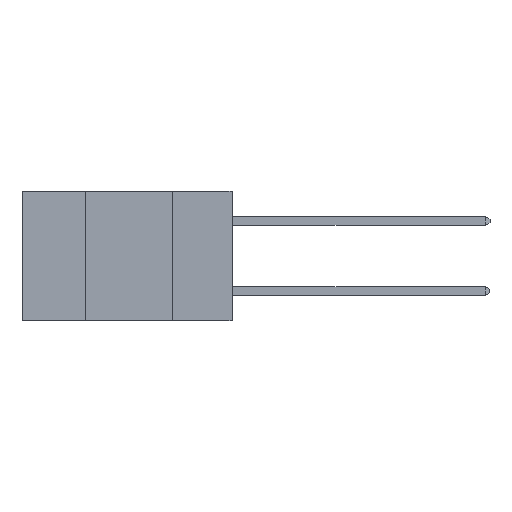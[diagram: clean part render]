
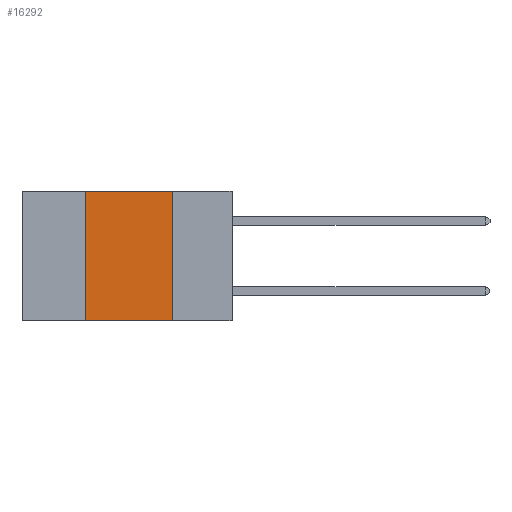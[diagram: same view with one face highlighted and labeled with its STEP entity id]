
A CAD part, left-side view. The second image highlights one B-rep face of the part: STEP entity #16292.
In plain terms, the highlighted planar face has unit normal (-1, 0, 0).
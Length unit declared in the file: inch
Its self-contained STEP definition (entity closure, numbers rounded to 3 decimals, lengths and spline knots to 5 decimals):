
#39 = CARTESIAN_POINT ( 'NONE',  ( 0., 0.17, 0. ) ) ;
#438 = FACE_OUTER_BOUND ( 'NONE', #10983, .T. ) ;
#834 = EDGE_CURVE ( 'NONE', #3131, #1718, #4436, .T. ) ;
#1718 = VERTEX_POINT ( 'NONE', #2014 ) ;
#2014 = CARTESIAN_POINT ( 'NONE',  ( 0., 0.17, -0.37 ) ) ;
#2199 = CARTESIAN_POINT ( 'NONE',  ( 0., 0.6, 0. ) ) ;
#3131 = VERTEX_POINT ( 'NONE', #10765 ) ;
#3248 = CARTESIAN_POINT ( 'NONE',  ( 0., 0.6, -0.37 ) ) ;
#3613 = DIRECTION ( 'NONE',  ( 0., 0., -1. ) ) ;
#3920 = VERTEX_POINT ( 'NONE', #12405 ) ;
#4272 = CARTESIAN_POINT ( 'NONE',  ( 0., 0.42, 0. ) ) ;
#4436 = LINE ( 'NONE', #3248, #14117 ) ;
#5239 = ORIENTED_EDGE ( 'NONE', *, *, #14721, .F. ) ;
#5408 = ORIENTED_EDGE ( 'NONE', *, *, #7624, .F. ) ;
#5524 = ORIENTED_EDGE ( 'NONE', *, *, #10147, .F. ) ;
#5672 = LINE ( 'NONE', #13204, #11907 ) ;
#5674 = DIRECTION ( 'NONE',  ( 0., 0., 1. ) ) ;
#5677 = ORIENTED_EDGE ( 'NONE', *, *, #834, .T. ) ;
#5875 = VECTOR ( 'NONE', #13056, 39.37008 ) ;
#7119 = LINE ( 'NONE', #4272, #13231 ) ;
#7591 = CARTESIAN_POINT ( 'NONE',  ( 0., 0.42, 0. ) ) ;
#7624 = EDGE_CURVE ( 'NONE', #15015, #3920, #5672, .T. ) ;
#8401 = AXIS2_PLACEMENT_3D ( 'NONE', #2199, #11319, #3613 ) ;
#8916 = PLANE ( 'NONE',  #8401 ) ;
#9879 = DIRECTION ( 'NONE',  ( 0., -1., 0. ) ) ;
#10147 = EDGE_CURVE ( 'NONE', #3131, #15015, #7119, .T. ) ;
#10765 = CARTESIAN_POINT ( 'NONE',  ( 0., 0.42, -0.37 ) ) ;
#10779 = DIRECTION ( 'NONE',  ( 0., -1., 0. ) ) ;
#10983 = EDGE_LOOP ( 'NONE', ( #5239, #5408, #5524, #5677 ) ) ;
#11319 = DIRECTION ( 'NONE',  ( 1., 0., 0. ) ) ;
#11907 = VECTOR ( 'NONE', #10779, 39.37008 ) ;
#12405 = CARTESIAN_POINT ( 'NONE',  ( 0., 0.17, 0. ) ) ;
#13056 = DIRECTION ( 'NONE',  ( 0., 0., -1. ) ) ;
#13204 = CARTESIAN_POINT ( 'NONE',  ( 0., 0.6, 0. ) ) ;
#13231 = VECTOR ( 'NONE', #5674, 39.37008 ) ;
#14117 = VECTOR ( 'NONE', #9879, 39.37008 ) ;
#14721 = EDGE_CURVE ( 'NONE', #3920, #1718, #15810, .T. ) ;
#15015 = VERTEX_POINT ( 'NONE', #7591 ) ;
#15810 = LINE ( 'NONE', #39, #5875 ) ;
#16292 = ADVANCED_FACE ( 'NONE', ( #438 ), #8916, .F. ) ;
